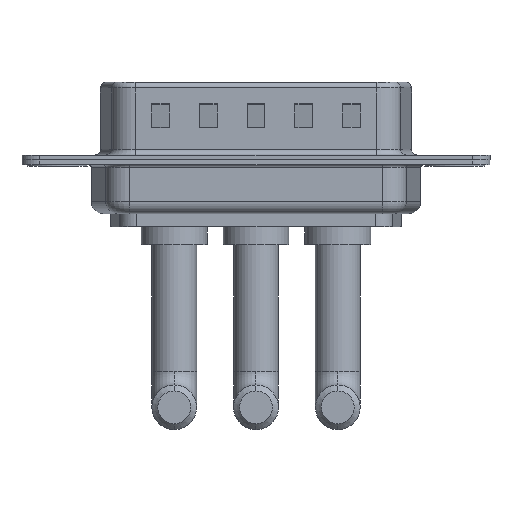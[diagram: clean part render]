
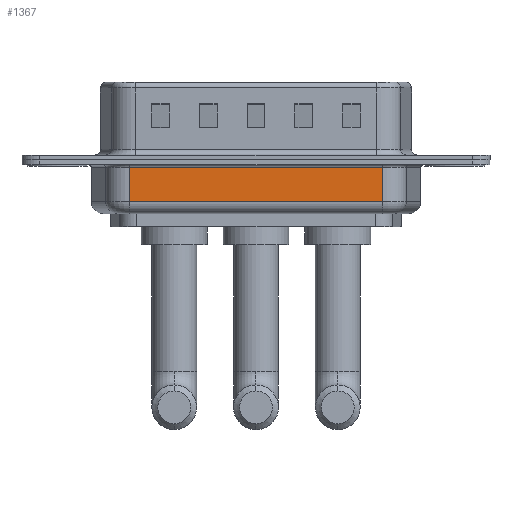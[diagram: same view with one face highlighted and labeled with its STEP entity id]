
A CAD part, front view. The second image highlights one B-rep face of the part: STEP entity #1367.
In plain terms, the highlighted planar face has unit normal (0, -1, 0).
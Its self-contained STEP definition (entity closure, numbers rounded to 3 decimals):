
#18 = EDGE_CURVE ( 'NONE', #10286, #7413, #11394, .T. ) ;
#1017 = FACE_OUTER_BOUND ( 'NONE', #11096, .T. ) ;
#1361 = ORIENTED_EDGE ( 'NONE', *, *, #18, .F. ) ;
#1367 = ADVANCED_FACE ( 'NONE', ( #1017 ), #4302, .F. ) ;
#1401 = CARTESIAN_POINT ( 'NONE',  ( 6.031, -5.35, -0.65 ) ) ;
#2151 = EDGE_CURVE ( 'NONE', #8250, #7413, #9099, .T. ) ;
#2350 = CARTESIAN_POINT ( 'NONE',  ( 27.269, -5.35, -3.5 ) ) ;
#2865 = CARTESIAN_POINT ( 'NONE',  ( 6.031, -5.35, -3.5 ) ) ;
#2907 = DIRECTION ( 'NONE',  ( 0., 0., 1. ) ) ;
#3251 = DIRECTION ( 'NONE',  ( 0., 1., 0. ) ) ;
#3304 = CARTESIAN_POINT ( 'NONE',  ( 27.269, -5.35, -0.65 ) ) ;
#3816 = DIRECTION ( 'NONE',  ( 0., 0., 1. ) ) ;
#3938 = EDGE_CURVE ( 'NONE', #5936, #8250, #6066, .T. ) ;
#4283 = AXIS2_PLACEMENT_3D ( 'NONE', #8586, #3251, #12949 ) ;
#4302 = PLANE ( 'NONE',  #4283 ) ;
#5922 = CARTESIAN_POINT ( 'NONE',  ( 6.031, -5.35, -3.5 ) ) ;
#5934 = ORIENTED_EDGE ( 'NONE', *, *, #6074, .T. ) ;
#5936 = VERTEX_POINT ( 'NONE', #2350 ) ;
#6066 = LINE ( 'NONE', #9149, #9513 ) ;
#6074 = EDGE_CURVE ( 'NONE', #10286, #5936, #7679, .T. ) ;
#6110 = ORIENTED_EDGE ( 'NONE', *, *, #3938, .T. ) ;
#6313 = ORIENTED_EDGE ( 'NONE', *, *, #2151, .T. ) ;
#7413 = VERTEX_POINT ( 'NONE', #1401 ) ;
#7679 = LINE ( 'NONE', #5922, #13822 ) ;
#8250 = VERTEX_POINT ( 'NONE', #3304 ) ;
#8586 = CARTESIAN_POINT ( 'NONE',  ( 6.031, -5.35, -4.5 ) ) ;
#8964 = CARTESIAN_POINT ( 'NONE',  ( 6.031, -5.35, -0.65 ) ) ;
#9099 = LINE ( 'NONE', #8964, #11699 ) ;
#9149 = CARTESIAN_POINT ( 'NONE',  ( 27.269, -5.35, -4.5 ) ) ;
#9513 = VECTOR ( 'NONE', #3816, 1000. ) ;
#10286 = VERTEX_POINT ( 'NONE', #2865 ) ;
#11096 = EDGE_LOOP ( 'NONE', ( #1361, #5934, #6110, #6313 ) ) ;
#11394 = LINE ( 'NONE', #12521, #12096 ) ;
#11396 = DIRECTION ( 'NONE',  ( 1., 0., 0. ) ) ;
#11699 = VECTOR ( 'NONE', #12195, 1000. ) ;
#12096 = VECTOR ( 'NONE', #2907, 1000. ) ;
#12195 = DIRECTION ( 'NONE',  ( -1., 0., 0. ) ) ;
#12521 = CARTESIAN_POINT ( 'NONE',  ( 6.031, -5.35, -4.5 ) ) ;
#12949 = DIRECTION ( 'NONE',  ( 0., 0., 1. ) ) ;
#13822 = VECTOR ( 'NONE', #11396, 1000. ) ;
